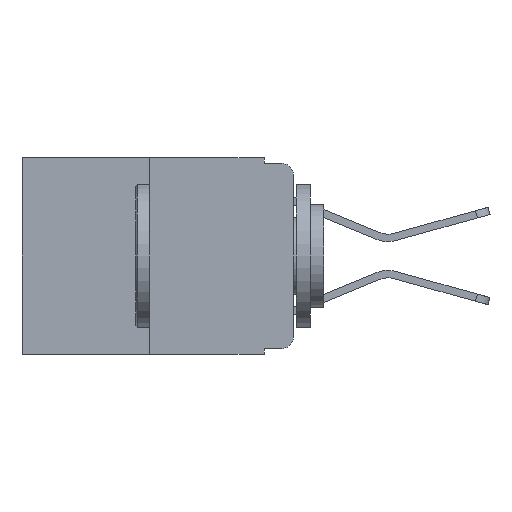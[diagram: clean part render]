
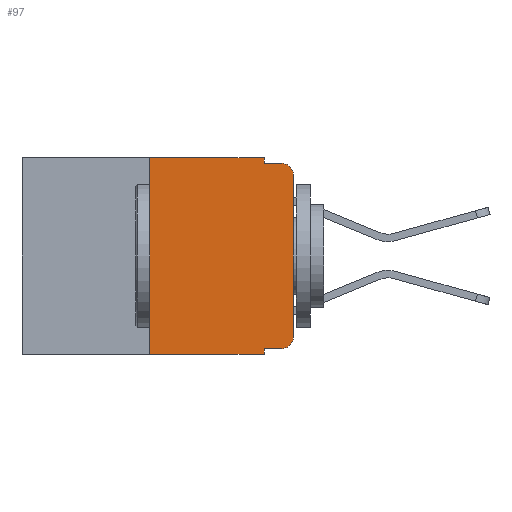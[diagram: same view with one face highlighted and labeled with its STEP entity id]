
A CAD part, left-side view. The second image highlights one B-rep face of the part: STEP entity #97.
In plain terms, the highlighted planar face has unit normal (-1, 0, 0).
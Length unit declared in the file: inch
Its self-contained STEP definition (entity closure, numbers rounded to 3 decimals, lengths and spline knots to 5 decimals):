
#97 = ADVANCED_FACE ( 'NONE', ( #14952 ), #5316, .F. ) ;
#303 = CARTESIAN_POINT ( 'NONE',  ( 0., 0.02, -0.01 ) ) ;
#911 = EDGE_CURVE ( 'NONE', #13191, #22431, #22266, .T. ) ;
#921 = CARTESIAN_POINT ( 'NONE',  ( 0., 0.473, 0. ) ) ;
#1416 = VERTEX_POINT ( 'NONE', #8264 ) ;
#1484 = EDGE_CURVE ( 'NONE', #22431, #9932, #10411, .T. ) ;
#1826 = DIRECTION ( 'NONE',  ( -1., 0., 0. ) ) ;
#2488 = CARTESIAN_POINT ( 'NONE',  ( 0., 0., 0. ) ) ;
#2667 = CARTESIAN_POINT ( 'NONE',  ( 0., 0.473, -0.343 ) ) ;
#2787 = CARTESIAN_POINT ( 'NONE',  ( 0., 0., -0.03 ) ) ;
#2897 = EDGE_CURVE ( 'NONE', #1416, #13191, #20779, .T. ) ;
#3030 = VERTEX_POINT ( 'NONE', #8840 ) ;
#3150 = VERTEX_POINT ( 'NONE', #303 ) ;
#3604 = EDGE_CURVE ( 'NONE', #1416, #3030, #7623, .T. ) ;
#3915 = VECTOR ( 'NONE', #21759, 39.37008 ) ;
#4148 = CARTESIAN_POINT ( 'NONE',  ( 0., 0.25, 0. ) ) ;
#4439 = ORIENTED_EDGE ( 'NONE', *, *, #14718, .T. ) ;
#4489 = CARTESIAN_POINT ( 'NONE',  ( 0., 0.051, 0. ) ) ;
#4683 = DIRECTION ( 'NONE',  ( 0., -1., 0. ) ) ;
#5079 = ORIENTED_EDGE ( 'NONE', *, *, #19806, .T. ) ;
#5316 = PLANE ( 'NONE',  #20589 ) ;
#5683 = EDGE_CURVE ( 'NONE', #11140, #3030, #6655, .T. ) ;
#6655 = LINE ( 'NONE', #20574, #21288 ) ;
#6678 = CARTESIAN_POINT ( 'NONE',  ( 0., 0.02, -0.313 ) ) ;
#6700 = CIRCLE ( 'NONE', #22162, 0.02 ) ;
#7264 = ORIENTED_EDGE ( 'NONE', *, *, #2897, .F. ) ;
#7623 = LINE ( 'NONE', #2667, #22170 ) ;
#7798 = VECTOR ( 'NONE', #19928, 39.37008 ) ;
#7863 = CARTESIAN_POINT ( 'NONE',  ( 0., 0.051, -0.333 ) ) ;
#8264 = CARTESIAN_POINT ( 'NONE',  ( 0., 0.25, -0.343 ) ) ;
#8630 = LINE ( 'NONE', #16069, #3915 ) ;
#8672 = DIRECTION ( 'NONE',  ( 0., 0., -1. ) ) ;
#8725 = DIRECTION ( 'NONE',  ( 0., -1., 0. ) ) ;
#8788 = EDGE_LOOP ( 'NONE', ( #18345, #8797, #19514, #25014, #16247, #7264, #17463, #23026, #4439, #5079 ) ) ;
#8797 = ORIENTED_EDGE ( 'NONE', *, *, #15211, .T. ) ;
#8840 = CARTESIAN_POINT ( 'NONE',  ( 0., 0.051, -0.343 ) ) ;
#8953 = DIRECTION ( 'NONE',  ( 0., 0., 1. ) ) ;
#9932 = VERTEX_POINT ( 'NONE', #22600 ) ;
#10411 = LINE ( 'NONE', #15860, #24827 ) ;
#10533 = DIRECTION ( 'NONE',  ( 0., -1., 0. ) ) ;
#10685 = VECTOR ( 'NONE', #8953, 39.37008 ) ;
#11140 = VERTEX_POINT ( 'NONE', #7863 ) ;
#11406 = EDGE_CURVE ( 'NONE', #15966, #16095, #23507, .T. ) ;
#12258 = CARTESIAN_POINT ( 'NONE',  ( 0., 0.473, 0. ) ) ;
#12299 = CARTESIAN_POINT ( 'NONE',  ( 0., 0., -0.313 ) ) ;
#13022 = DIRECTION ( 'NONE',  ( 0., 0., -1. ) ) ;
#13055 = DIRECTION ( 'NONE',  ( 1., 0., 0. ) ) ;
#13191 = VERTEX_POINT ( 'NONE', #21558 ) ;
#13670 = CARTESIAN_POINT ( 'NONE',  ( 0., 0.02, -0.03 ) ) ;
#14718 = EDGE_CURVE ( 'NONE', #11140, #15585, #8630, .T. ) ;
#14952 = FACE_OUTER_BOUND ( 'NONE', #8788, .T. ) ;
#15211 = EDGE_CURVE ( 'NONE', #16095, #3150, #23115, .T. ) ;
#15585 = VERTEX_POINT ( 'NONE', #18514 ) ;
#15607 = DIRECTION ( 'NONE',  ( 0., 0., -1. ) ) ;
#15813 = DIRECTION ( 'NONE',  ( 0., 0., -1. ) ) ;
#15860 = CARTESIAN_POINT ( 'NONE',  ( 0., 0.051, 0. ) ) ;
#15966 = VERTEX_POINT ( 'NONE', #12299 ) ;
#16069 = CARTESIAN_POINT ( 'NONE',  ( 0., 0.051, -0.333 ) ) ;
#16095 = VERTEX_POINT ( 'NONE', #2787 ) ;
#16247 = ORIENTED_EDGE ( 'NONE', *, *, #911, .F. ) ;
#17356 = VECTOR ( 'NONE', #10533, 39.37008 ) ;
#17463 = ORIENTED_EDGE ( 'NONE', *, *, #3604, .T. ) ;
#17754 = EDGE_CURVE ( 'NONE', #9932, #3150, #22320, .T. ) ;
#18011 = AXIS2_PLACEMENT_3D ( 'NONE', #13670, #1826, #15607 ) ;
#18345 = ORIENTED_EDGE ( 'NONE', *, *, #11406, .T. ) ;
#18514 = CARTESIAN_POINT ( 'NONE',  ( 0., 0.02, -0.333 ) ) ;
#18691 = DIRECTION ( 'NONE',  ( 0., 0., -1. ) ) ;
#19514 = ORIENTED_EDGE ( 'NONE', *, *, #17754, .F. ) ;
#19806 = EDGE_CURVE ( 'NONE', #15585, #15966, #6700, .T. ) ;
#19928 = DIRECTION ( 'NONE',  ( 0., 0., 1. ) ) ;
#20043 = DIRECTION ( 'NONE',  ( -1., 0., 0. ) ) ;
#20574 = CARTESIAN_POINT ( 'NONE',  ( 0., 0.051, 0. ) ) ;
#20589 = AXIS2_PLACEMENT_3D ( 'NONE', #12258, #13055, #13022 ) ;
#20779 = LINE ( 'NONE', #4148, #10685 ) ;
#21122 = VECTOR ( 'NONE', #8725, 39.37008 ) ;
#21288 = VECTOR ( 'NONE', #18691, 39.37008 ) ;
#21558 = CARTESIAN_POINT ( 'NONE',  ( 0., 0.25, 0. ) ) ;
#21759 = DIRECTION ( 'NONE',  ( 0., -1., 0. ) ) ;
#22162 = AXIS2_PLACEMENT_3D ( 'NONE', #6678, #20043, #8672 ) ;
#22170 = VECTOR ( 'NONE', #4683, 39.37008 ) ;
#22266 = LINE ( 'NONE', #921, #21122 ) ;
#22320 = LINE ( 'NONE', #23726, #17356 ) ;
#22431 = VERTEX_POINT ( 'NONE', #4489 ) ;
#22600 = CARTESIAN_POINT ( 'NONE',  ( 0., 0.051, -0.01 ) ) ;
#23026 = ORIENTED_EDGE ( 'NONE', *, *, #5683, .F. ) ;
#23115 = CIRCLE ( 'NONE', #18011, 0.02 ) ;
#23507 = LINE ( 'NONE', #2488, #7798 ) ;
#23726 = CARTESIAN_POINT ( 'NONE',  ( 0., 0.051, -0.01 ) ) ;
#24827 = VECTOR ( 'NONE', #15813, 39.37008 ) ;
#25014 = ORIENTED_EDGE ( 'NONE', *, *, #1484, .F. ) ;
